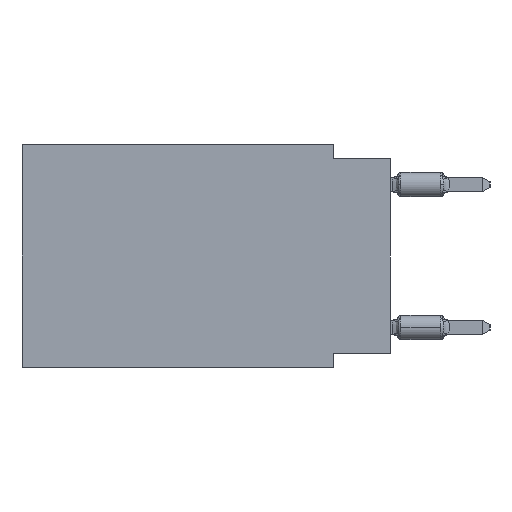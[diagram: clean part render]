
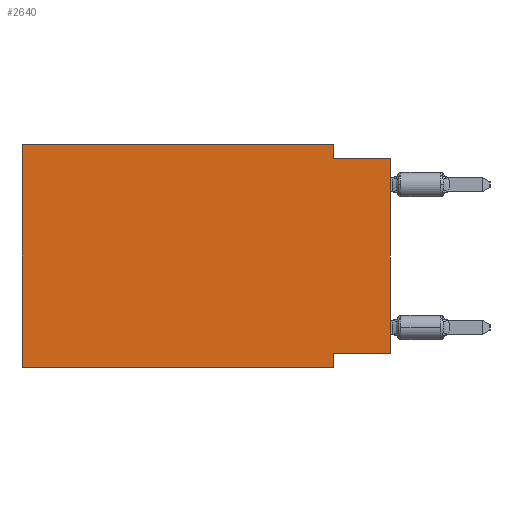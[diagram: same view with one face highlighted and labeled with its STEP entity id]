
A CAD part, left-side view. The second image highlights one B-rep face of the part: STEP entity #2640.
In plain terms, the highlighted planar face has unit normal (-1, 0, 0).
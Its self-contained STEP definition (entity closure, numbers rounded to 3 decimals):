
#546 = EDGE_CURVE ( 'NONE', #37939, #7431, #24894, .T. ) ;
#1046 = VECTOR ( 'NONE', #11705, 1000. ) ;
#1331 = ORIENTED_EDGE ( 'NONE', *, *, #30152, .F. ) ;
#2413 = CARTESIAN_POINT ( 'NONE',  ( 0., 16.383, 0. ) ) ;
#2445 = VERTEX_POINT ( 'NONE', #10709 ) ;
#2640 = ADVANCED_FACE ( 'NONE', ( #40560 ), #11954, .F. ) ;
#3061 = CARTESIAN_POINT ( 'NONE',  ( 0., 0., -9.271 ) ) ;
#4220 = ORIENTED_EDGE ( 'NONE', *, *, #27433, .T. ) ;
#4221 = VECTOR ( 'NONE', #27945, 1000. ) ;
#4854 = EDGE_CURVE ( 'NONE', #19187, #27061, #22030, .T. ) ;
#4856 = DIRECTION ( 'NONE',  ( 0., -1., 0. ) ) ;
#6068 = CARTESIAN_POINT ( 'NONE',  ( 0., 2.54, 0. ) ) ;
#6662 = VECTOR ( 'NONE', #4856, 1000. ) ;
#7323 = CARTESIAN_POINT ( 'NONE',  ( 0., 0., -0.635 ) ) ;
#7431 = VERTEX_POINT ( 'NONE', #15658 ) ;
#7693 = VECTOR ( 'NONE', #24535, 1000. ) ;
#9285 = LINE ( 'NONE', #40811, #4221 ) ;
#9944 = ORIENTED_EDGE ( 'NONE', *, *, #546, .T. ) ;
#10709 = CARTESIAN_POINT ( 'NONE',  ( 0., 2.54, -9.271 ) ) ;
#10970 = VERTEX_POINT ( 'NONE', #7323 ) ;
#11705 = DIRECTION ( 'NONE',  ( 0., -1., 0. ) ) ;
#11771 = ORIENTED_EDGE ( 'NONE', *, *, #14727, .F. ) ;
#11954 = PLANE ( 'NONE',  #21514 ) ;
#13264 = DIRECTION ( 'NONE',  ( 0., 0., -1. ) ) ;
#14727 = EDGE_CURVE ( 'NONE', #15824, #2445, #24844, .T. ) ;
#15031 = ORIENTED_EDGE ( 'NONE', *, *, #4854, .F. ) ;
#15658 = CARTESIAN_POINT ( 'NONE',  ( 0., 2.54, -9.906 ) ) ;
#15824 = VERTEX_POINT ( 'NONE', #30083 ) ;
#16630 = EDGE_LOOP ( 'NONE', ( #4220, #16914, #15031, #18358, #1331, #9944, #27154, #11771 ) ) ;
#16914 = ORIENTED_EDGE ( 'NONE', *, *, #21964, .F. ) ;
#17214 = CARTESIAN_POINT ( 'NONE',  ( 0., 2.54, 0. ) ) ;
#17240 = EDGE_CURVE ( 'NONE', #27896, #19187, #23737, .T. ) ;
#18358 = ORIENTED_EDGE ( 'NONE', *, *, #17240, .F. ) ;
#19187 = VERTEX_POINT ( 'NONE', #17214 ) ;
#21514 = AXIS2_PLACEMENT_3D ( 'NONE', #2413, #30810, #24605 ) ;
#21750 = CARTESIAN_POINT ( 'NONE',  ( 0., 16.383, 0. ) ) ;
#21964 = EDGE_CURVE ( 'NONE', #27061, #10970, #24364, .T. ) ;
#22030 = LINE ( 'NONE', #6068, #7693 ) ;
#23498 = VECTOR ( 'NONE', #25273, 1000. ) ;
#23737 = LINE ( 'NONE', #33251, #6662 ) ;
#23825 = VECTOR ( 'NONE', #30847, 1000. ) ;
#24364 = LINE ( 'NONE', #40115, #1046 ) ;
#24535 = DIRECTION ( 'NONE',  ( 0., 0., -1. ) ) ;
#24605 = DIRECTION ( 'NONE',  ( 0., 0., -1. ) ) ;
#24844 = LINE ( 'NONE', #3061, #23825 ) ;
#24894 = LINE ( 'NONE', #34837, #26652 ) ;
#25273 = DIRECTION ( 'NONE',  ( 0., 0., 1. ) ) ;
#26652 = VECTOR ( 'NONE', #31506, 1000. ) ;
#27061 = VERTEX_POINT ( 'NONE', #39047 ) ;
#27154 = ORIENTED_EDGE ( 'NONE', *, *, #32410, .F. ) ;
#27433 = EDGE_CURVE ( 'NONE', #15824, #10970, #9285, .T. ) ;
#27896 = VERTEX_POINT ( 'NONE', #39067 ) ;
#27945 = DIRECTION ( 'NONE',  ( 0., 0., 1. ) ) ;
#29418 = LINE ( 'NONE', #32945, #40234 ) ;
#30083 = CARTESIAN_POINT ( 'NONE',  ( 0., 0., -9.271 ) ) ;
#30152 = EDGE_CURVE ( 'NONE', #37939, #27896, #37710, .T. ) ;
#30810 = DIRECTION ( 'NONE',  ( 1., 0., 0. ) ) ;
#30847 = DIRECTION ( 'NONE',  ( 0., 1., 0. ) ) ;
#31506 = DIRECTION ( 'NONE',  ( 0., -1., 0. ) ) ;
#32410 = EDGE_CURVE ( 'NONE', #2445, #7431, #29418, .T. ) ;
#32945 = CARTESIAN_POINT ( 'NONE',  ( 0., 2.54, -9.906 ) ) ;
#33251 = CARTESIAN_POINT ( 'NONE',  ( 0., 16.383, 0. ) ) ;
#34837 = CARTESIAN_POINT ( 'NONE',  ( 0., 16.383, -9.906 ) ) ;
#37710 = LINE ( 'NONE', #21750, #23498 ) ;
#37723 = CARTESIAN_POINT ( 'NONE',  ( 0., 16.383, -9.906 ) ) ;
#37939 = VERTEX_POINT ( 'NONE', #37723 ) ;
#39047 = CARTESIAN_POINT ( 'NONE',  ( 0., 2.54, -0.635 ) ) ;
#39067 = CARTESIAN_POINT ( 'NONE',  ( 0., 16.383, 0. ) ) ;
#40115 = CARTESIAN_POINT ( 'NONE',  ( 0., 0., -0.635 ) ) ;
#40234 = VECTOR ( 'NONE', #13264, 1000. ) ;
#40560 = FACE_OUTER_BOUND ( 'NONE', #16630, .T. ) ;
#40811 = CARTESIAN_POINT ( 'NONE',  ( 0., 0., 0. ) ) ;
